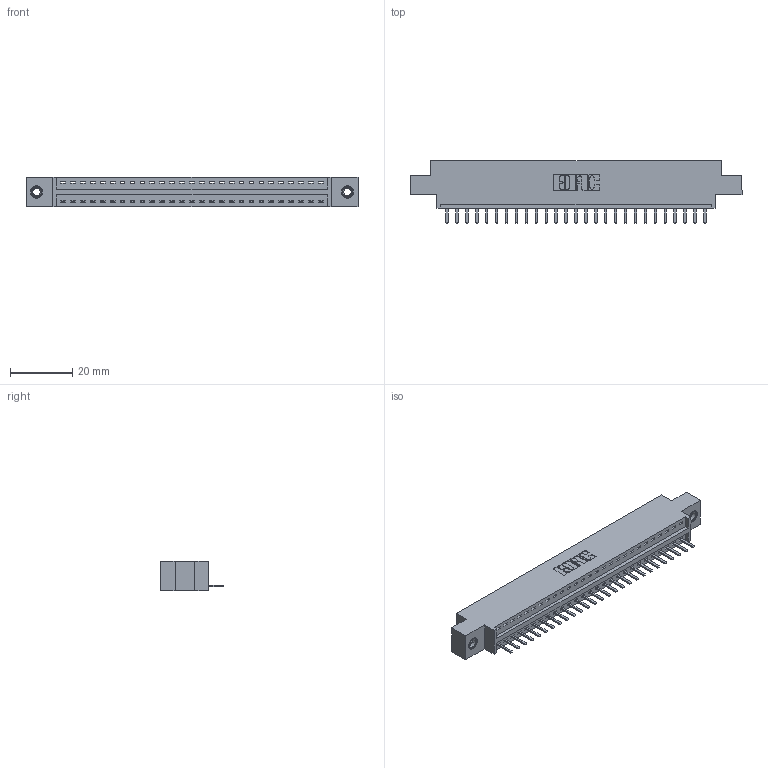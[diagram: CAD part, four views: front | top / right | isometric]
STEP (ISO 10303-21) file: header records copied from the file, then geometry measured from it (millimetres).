
FILE_DESCRIPTION (( 'STEP AP203' ), '1' );
FILE_NAME ('346-027-520-607.STEP', '2022-05-06T04:08:44', ( '' ), ( '' ), 'SwSTEP 2.0', 'SolidWorks 2020', '' );
FILE_SCHEMA (( 'CONFIG_CONTROL_DESIGN' ));
Length unit declared in the file: inch
Products named in the file (4): 345-292-001_345-293-120; 345-250-001_345-250-005-103; 346-027-520-607; 346 Part_0.170 Offset - 0.156 Dia-TI
Assembly tree (30 placements, depth 2):
  346-027-520-607
    346 Part_0.170 Offset - 0.156 Dia-TI
    345-292-001_345-293-120  x27
    345-250-001_345-250-005-103  x2
Bounding box: 106.3 x 20.02 x 9.4 mm (x, y, z)
Volume: 9826 mm3; surface area: 12055.1 mm2
Topology: 30 solids, 30 shells, 1860 faces, 5445 edges, 3550 vertices
Faces by surface type: plane 1246, cylinder 598, cone 12, torus 4
Entity records: 20208 total; most frequent: CARTESIAN_POINT 3464, ORIENTED_EDGE 3406, DIRECTION 3087, EDGE_CURVE 1703, LINE 1439, VECTOR 1439, VERTEX_POINT 1128, AXIS2_PLACEMENT_3D 824
